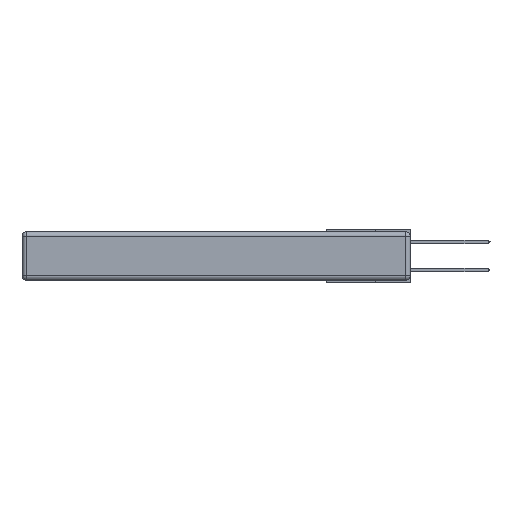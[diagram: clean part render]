
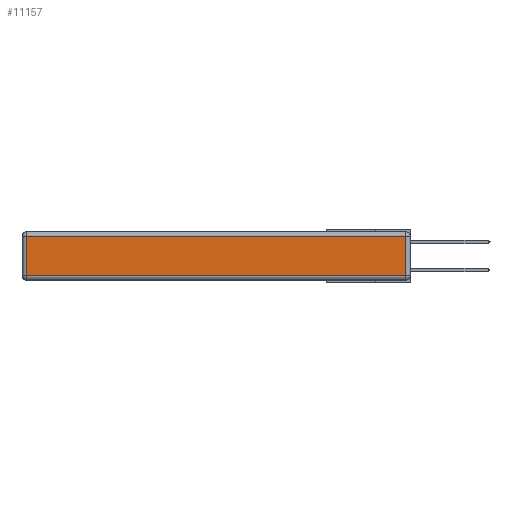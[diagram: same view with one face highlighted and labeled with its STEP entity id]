
A CAD part, left-side view. The second image highlights one B-rep face of the part: STEP entity #11157.
In plain terms, the highlighted planar face has unit normal (-1, 0, 0).
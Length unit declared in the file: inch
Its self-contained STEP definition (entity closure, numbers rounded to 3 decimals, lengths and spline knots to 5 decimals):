
#194 = CARTESIAN_POINT ( 'NONE',  ( 0., 2.72, -0.313 ) ) ;
#206 = VERTEX_POINT ( 'NONE', #194 ) ;
#216 = DIRECTION ( 'NONE',  ( 0., 0., -1. ) ) ;
#833 = ORIENTED_EDGE ( 'NONE', *, *, #23042, .T. ) ;
#1062 = FACE_OUTER_BOUND ( 'NONE', #9903, .T. ) ;
#1782 = DIRECTION ( 'NONE',  ( 0., 0., 1. ) ) ;
#4972 = LINE ( 'NONE', #9176, #9265 ) ;
#5499 = CARTESIAN_POINT ( 'NONE',  ( 0., 0.03, -0.313 ) ) ;
#6111 = EDGE_CURVE ( 'NONE', #6150, #13634, #4972, .T. ) ;
#6150 = VERTEX_POINT ( 'NONE', #5499 ) ;
#6357 = CARTESIAN_POINT ( 'NONE',  ( 0., 2.72, -0.03 ) ) ;
#6476 = ORIENTED_EDGE ( 'NONE', *, *, #11513, .T. ) ;
#6502 = LINE ( 'NONE', #21098, #23108 ) ;
#7453 = CARTESIAN_POINT ( 'NONE',  ( 0., 2.72, -0.343 ) ) ;
#7944 = VECTOR ( 'NONE', #216, 39.37008 ) ;
#9176 = CARTESIAN_POINT ( 'NONE',  ( 0., 0.03, -0.343 ) ) ;
#9265 = VECTOR ( 'NONE', #1782, 39.37008 ) ;
#9284 = LINE ( 'NONE', #14831, #17278 ) ;
#9903 = EDGE_LOOP ( 'NONE', ( #6476, #20209, #833, #16216 ) ) ;
#10025 = DIRECTION ( 'NONE',  ( 0., 0., 1. ) ) ;
#11157 = ADVANCED_FACE ( 'NONE', ( #1062 ), #22499, .T. ) ;
#11351 = EDGE_CURVE ( 'NONE', #22248, #206, #16529, .T. ) ;
#11513 = EDGE_CURVE ( 'NONE', #206, #6150, #6502, .T. ) ;
#13632 = CARTESIAN_POINT ( 'NONE',  ( 0., 0., -0.343 ) ) ;
#13634 = VERTEX_POINT ( 'NONE', #19821 ) ;
#14831 = CARTESIAN_POINT ( 'NONE',  ( 0., 2.75, -0.03 ) ) ;
#16216 = ORIENTED_EDGE ( 'NONE', *, *, #11351, .T. ) ;
#16529 = LINE ( 'NONE', #7453, #7944 ) ;
#16561 = AXIS2_PLACEMENT_3D ( 'NONE', #13632, #19141, #10025 ) ;
#16662 = DIRECTION ( 'NONE',  ( 0., 1., 0. ) ) ;
#17278 = VECTOR ( 'NONE', #16662, 39.37008 ) ;
#19141 = DIRECTION ( 'NONE',  ( -1., 0., 0. ) ) ;
#19192 = DIRECTION ( 'NONE',  ( 0., -1., 0. ) ) ;
#19821 = CARTESIAN_POINT ( 'NONE',  ( 0., 0.03, -0.03 ) ) ;
#20209 = ORIENTED_EDGE ( 'NONE', *, *, #6111, .T. ) ;
#21098 = CARTESIAN_POINT ( 'NONE',  ( 0., 0., -0.313 ) ) ;
#22248 = VERTEX_POINT ( 'NONE', #6357 ) ;
#22499 = PLANE ( 'NONE',  #16561 ) ;
#23042 = EDGE_CURVE ( 'NONE', #13634, #22248, #9284, .T. ) ;
#23108 = VECTOR ( 'NONE', #19192, 39.37008 ) ;
